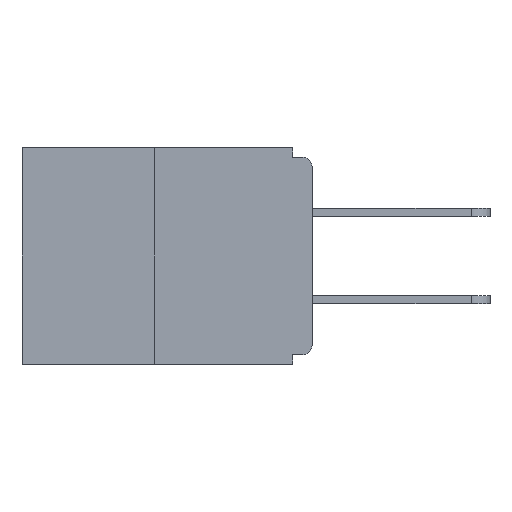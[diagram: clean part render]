
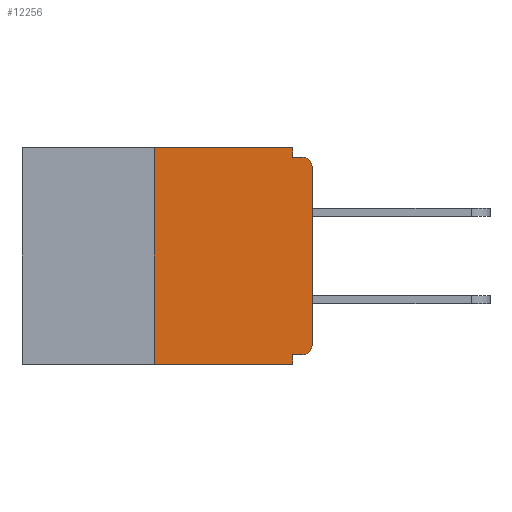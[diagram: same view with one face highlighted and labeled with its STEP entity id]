
A CAD part, left-side view. The second image highlights one B-rep face of the part: STEP entity #12256.
In plain terms, the highlighted planar face has unit normal (-1, 0, 0).
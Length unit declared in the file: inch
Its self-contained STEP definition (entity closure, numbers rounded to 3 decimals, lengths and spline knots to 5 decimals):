
#35 = EDGE_CURVE ( 'NONE', #8040, #4283, #9924, .T. ) ;
#152 = EDGE_CURVE ( 'NONE', #4144, #11577, #3746, .T. ) ;
#948 = VECTOR ( 'NONE', #12822, 39.37008 ) ;
#1049 = CIRCLE ( 'NONE', #2292, 0.015 ) ;
#1198 = DIRECTION ( 'NONE',  ( -1., 0., 0. ) ) ;
#1287 = VECTOR ( 'NONE', #8750, 39.37008 ) ;
#1558 = ORIENTED_EDGE ( 'NONE', *, *, #6423, .F. ) ;
#1632 = ORIENTED_EDGE ( 'NONE', *, *, #13754, .F. ) ;
#1784 = CARTESIAN_POINT ( 'NONE',  ( 0., 0., 0. ) ) ;
#2050 = ORIENTED_EDGE ( 'NONE', *, *, #12734, .T. ) ;
#2272 = DIRECTION ( 'NONE',  ( 0., 0., -1. ) ) ;
#2292 = AXIS2_PLACEMENT_3D ( 'NONE', #8478, #1198, #7285 ) ;
#2399 = VECTOR ( 'NONE', #13588, 39.37008 ) ;
#2488 = CARTESIAN_POINT ( 'NONE',  ( 0., 0.015, -0.015 ) ) ;
#3090 = CARTESIAN_POINT ( 'NONE',  ( 0., 0.25, 0. ) ) ;
#3159 = DIRECTION ( 'NONE',  ( 0., -1., 0. ) ) ;
#3293 = CARTESIAN_POINT ( 'NONE',  ( 0., 0.46, 0. ) ) ;
#3356 = VECTOR ( 'NONE', #14248, 39.37008 ) ;
#3452 = DIRECTION ( 'NONE',  ( 0., 0., 1. ) ) ;
#3464 = CARTESIAN_POINT ( 'NONE',  ( 0., 0.46, 0. ) ) ;
#3618 = DIRECTION ( 'NONE',  ( 1., 0., 0. ) ) ;
#3739 = VERTEX_POINT ( 'NONE', #2488 ) ;
#3746 = LINE ( 'NONE', #15669, #2399 ) ;
#4144 = VERTEX_POINT ( 'NONE', #14884 ) ;
#4229 = LINE ( 'NONE', #10296, #948 ) ;
#4283 = VERTEX_POINT ( 'NONE', #3090 ) ;
#4734 = PLANE ( 'NONE',  #15771 ) ;
#6143 = ORIENTED_EDGE ( 'NONE', *, *, #12372, .T. ) ;
#6423 = EDGE_CURVE ( 'NONE', #4283, #15693, #14941, .T. ) ;
#6484 = ORIENTED_EDGE ( 'NONE', *, *, #11013, .T. ) ;
#6567 = EDGE_LOOP ( 'NONE', ( #1558, #12818, #6484, #1632, #14376, #6143, #2050, #14471, #8926, #6859 ) ) ;
#6693 = VERTEX_POINT ( 'NONE', #12240 ) ;
#6735 = AXIS2_PLACEMENT_3D ( 'NONE', #9364, #15546, #11849 ) ;
#6852 = CARTESIAN_POINT ( 'NONE',  ( 0., 0.25, 0. ) ) ;
#6859 = ORIENTED_EDGE ( 'NONE', *, *, #9392, .F. ) ;
#7285 = DIRECTION ( 'NONE',  ( 0., 0., -1. ) ) ;
#7316 = LINE ( 'NONE', #14863, #11599 ) ;
#7499 = CARTESIAN_POINT ( 'NONE',  ( 0., 0.46, -0.343 ) ) ;
#7753 = EDGE_CURVE ( 'NONE', #11089, #3739, #11243, .T. ) ;
#8040 = VERTEX_POINT ( 'NONE', #12342 ) ;
#8478 = CARTESIAN_POINT ( 'NONE',  ( 0., 0.015, -0.313 ) ) ;
#8490 = VERTEX_POINT ( 'NONE', #8742 ) ;
#8742 = CARTESIAN_POINT ( 'NONE',  ( 0., 0., -0.313 ) ) ;
#8750 = DIRECTION ( 'NONE',  ( 0., -1., 0. ) ) ;
#8926 = ORIENTED_EDGE ( 'NONE', *, *, #11570, .F. ) ;
#8929 = VECTOR ( 'NONE', #3452, 39.37008 ) ;
#9364 = CARTESIAN_POINT ( 'NONE',  ( 0., 0.015, -0.03 ) ) ;
#9392 = EDGE_CURVE ( 'NONE', #15693, #6693, #4229, .T. ) ;
#9675 = CARTESIAN_POINT ( 'NONE',  ( 0., 0.031, -0.343 ) ) ;
#9924 = LINE ( 'NONE', #6852, #8929 ) ;
#10296 = CARTESIAN_POINT ( 'NONE',  ( 0., 0.031, 0. ) ) ;
#10891 = VECTOR ( 'NONE', #14622, 39.37008 ) ;
#11013 = EDGE_CURVE ( 'NONE', #8040, #15759, #14377, .T. ) ;
#11089 = VERTEX_POINT ( 'NONE', #13319 ) ;
#11243 = CIRCLE ( 'NONE', #6735, 0.015 ) ;
#11281 = LINE ( 'NONE', #15558, #13597 ) ;
#11453 = FACE_OUTER_BOUND ( 'NONE', #6567, .T. ) ;
#11570 = EDGE_CURVE ( 'NONE', #6693, #3739, #11281, .T. ) ;
#11577 = VERTEX_POINT ( 'NONE', #13095 ) ;
#11599 = VECTOR ( 'NONE', #12451, 39.37008 ) ;
#11849 = DIRECTION ( 'NONE',  ( 0., 0., -1. ) ) ;
#12240 = CARTESIAN_POINT ( 'NONE',  ( 0., 0.031, -0.015 ) ) ;
#12256 = ADVANCED_FACE ( 'NONE', ( #11453 ), #4734, .F. ) ;
#12342 = CARTESIAN_POINT ( 'NONE',  ( 0., 0.25, -0.343 ) ) ;
#12372 = EDGE_CURVE ( 'NONE', #4144, #8490, #1049, .T. ) ;
#12451 = DIRECTION ( 'NONE',  ( 0., 0., -1. ) ) ;
#12734 = EDGE_CURVE ( 'NONE', #8490, #11089, #14519, .T. ) ;
#12818 = ORIENTED_EDGE ( 'NONE', *, *, #35, .F. ) ;
#12822 = DIRECTION ( 'NONE',  ( 0., 0., -1. ) ) ;
#13095 = CARTESIAN_POINT ( 'NONE',  ( 0., 0.031, -0.328 ) ) ;
#13319 = CARTESIAN_POINT ( 'NONE',  ( 0., 0., -0.03 ) ) ;
#13588 = DIRECTION ( 'NONE',  ( 0., 1., 0. ) ) ;
#13597 = VECTOR ( 'NONE', #3159, 39.37008 ) ;
#13729 = CARTESIAN_POINT ( 'NONE',  ( 0., 0.031, 0. ) ) ;
#13754 = EDGE_CURVE ( 'NONE', #11577, #15759, #7316, .T. ) ;
#14248 = DIRECTION ( 'NONE',  ( 0., 0., 1. ) ) ;
#14376 = ORIENTED_EDGE ( 'NONE', *, *, #152, .F. ) ;
#14377 = LINE ( 'NONE', #7499, #1287 ) ;
#14471 = ORIENTED_EDGE ( 'NONE', *, *, #7753, .T. ) ;
#14519 = LINE ( 'NONE', #1784, #3356 ) ;
#14622 = DIRECTION ( 'NONE',  ( 0., -1., 0. ) ) ;
#14863 = CARTESIAN_POINT ( 'NONE',  ( 0., 0.031, -0.343 ) ) ;
#14884 = CARTESIAN_POINT ( 'NONE',  ( 0., 0.015, -0.328 ) ) ;
#14941 = LINE ( 'NONE', #3293, #10891 ) ;
#15546 = DIRECTION ( 'NONE',  ( -1., 0., 0. ) ) ;
#15558 = CARTESIAN_POINT ( 'NONE',  ( 0., 0., -0.015 ) ) ;
#15669 = CARTESIAN_POINT ( 'NONE',  ( 0., 0., -0.328 ) ) ;
#15693 = VERTEX_POINT ( 'NONE', #13729 ) ;
#15759 = VERTEX_POINT ( 'NONE', #9675 ) ;
#15771 = AXIS2_PLACEMENT_3D ( 'NONE', #3464, #3618, #2272 ) ;
